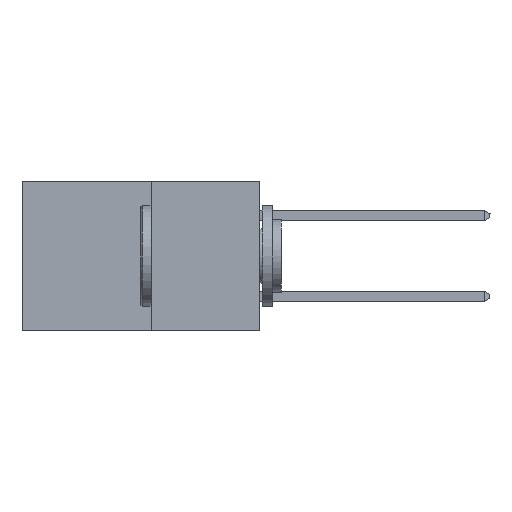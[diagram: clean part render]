
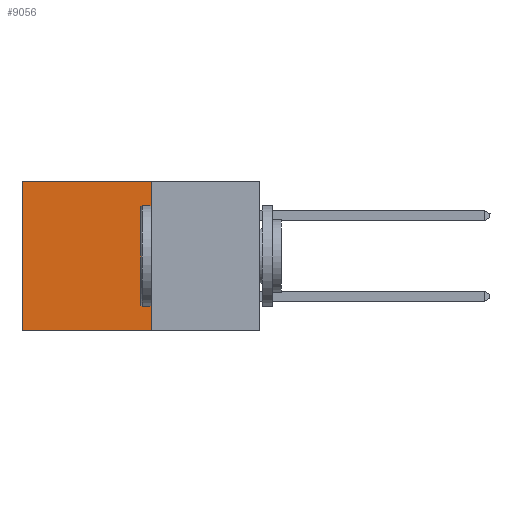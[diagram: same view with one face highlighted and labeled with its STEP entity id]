
A CAD part, left-side view. The second image highlights one B-rep face of the part: STEP entity #9056.
In plain terms, the highlighted planar face has unit normal (-1, 0, 0).
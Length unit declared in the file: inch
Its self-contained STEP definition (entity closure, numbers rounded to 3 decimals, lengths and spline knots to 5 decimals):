
#73 = PLANE ( 'NONE',  #2354 ) ;
#203 = CARTESIAN_POINT ( 'NONE',  ( 0.277, 0.59, -0.37 ) ) ;
#272 = VERTEX_POINT ( 'NONE', #12651 ) ;
#663 = LINE ( 'NONE', #12251, #3327 ) ;
#1080 = DIRECTION ( 'NONE',  ( 1., 0., 0. ) ) ;
#1155 = ORIENTED_EDGE ( 'NONE', *, *, #5273, .T. ) ;
#1808 = LINE ( 'NONE', #3978, #11651 ) ;
#2354 = AXIS2_PLACEMENT_3D ( 'NONE', #5108, #1080, #8077 ) ;
#3246 = VECTOR ( 'NONE', #10846, 39.37008 ) ;
#3327 = VECTOR ( 'NONE', #11333, 39.37008 ) ;
#3481 = LINE ( 'NONE', #8538, #8142 ) ;
#3509 = DIRECTION ( 'NONE',  ( 0., 0., -1. ) ) ;
#3867 = ORIENTED_EDGE ( 'NONE', *, *, #4024, .F. ) ;
#3978 = CARTESIAN_POINT ( 'NONE',  ( 0.277, 0.59, -0.37 ) ) ;
#4024 = EDGE_CURVE ( 'NONE', #272, #9190, #3481, .T. ) ;
#4790 = CARTESIAN_POINT ( 'NONE',  ( 0.277, 0.27, 0. ) ) ;
#5108 = CARTESIAN_POINT ( 'NONE',  ( 0.277, 0.27, -0.37 ) ) ;
#5273 = EDGE_CURVE ( 'NONE', #7480, #9190, #1808, .T. ) ;
#6500 = ORIENTED_EDGE ( 'NONE', *, *, #11302, .F. ) ;
#7047 = VERTEX_POINT ( 'NONE', #4790 ) ;
#7343 = FACE_OUTER_BOUND ( 'NONE', #9803, .T. ) ;
#7480 = VERTEX_POINT ( 'NONE', #11220 ) ;
#7565 = EDGE_CURVE ( 'NONE', #7047, #7480, #663, .T. ) ;
#8077 = DIRECTION ( 'NONE',  ( 0., 0., -1. ) ) ;
#8142 = VECTOR ( 'NONE', #8979, 39.37008 ) ;
#8538 = CARTESIAN_POINT ( 'NONE',  ( 0.277, 0.27, -0.37 ) ) ;
#8876 = LINE ( 'NONE', #9920, #3246 ) ;
#8979 = DIRECTION ( 'NONE',  ( 0., 1., 0. ) ) ;
#9056 = ADVANCED_FACE ( 'NONE', ( #7343 ), #73, .F. ) ;
#9162 = ORIENTED_EDGE ( 'NONE', *, *, #7565, .T. ) ;
#9190 = VERTEX_POINT ( 'NONE', #203 ) ;
#9803 = EDGE_LOOP ( 'NONE', ( #1155, #3867, #6500, #9162 ) ) ;
#9920 = CARTESIAN_POINT ( 'NONE',  ( 0.277, 0.27, -0.37 ) ) ;
#10846 = DIRECTION ( 'NONE',  ( 0., 0., -1. ) ) ;
#11220 = CARTESIAN_POINT ( 'NONE',  ( 0.277, 0.59, 0. ) ) ;
#11302 = EDGE_CURVE ( 'NONE', #7047, #272, #8876, .T. ) ;
#11333 = DIRECTION ( 'NONE',  ( 0., 1., 0. ) ) ;
#11651 = VECTOR ( 'NONE', #3509, 39.37008 ) ;
#12251 = CARTESIAN_POINT ( 'NONE',  ( 0.277, 0.27, 0. ) ) ;
#12651 = CARTESIAN_POINT ( 'NONE',  ( 0.277, 0.27, -0.37 ) ) ;
